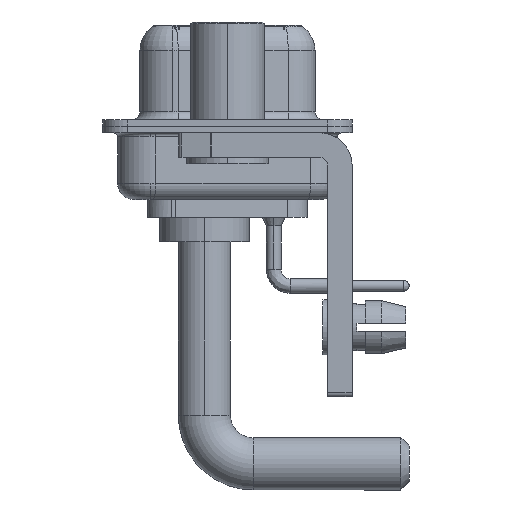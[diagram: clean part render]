
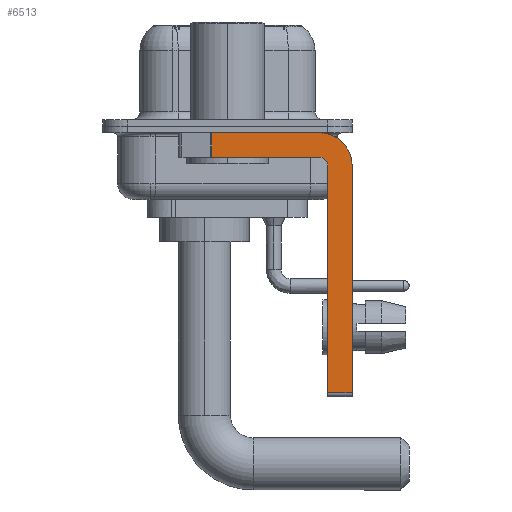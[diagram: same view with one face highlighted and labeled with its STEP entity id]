
A CAD part, left-side view. The second image highlights one B-rep face of the part: STEP entity #6513.
In plain terms, the highlighted planar face has unit normal (-1, 0, 0).
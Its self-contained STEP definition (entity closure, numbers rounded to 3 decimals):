
#29 = EDGE_CURVE ( 'NONE', #12476, #24220, #2890, .T. ) ;
#83 = DIRECTION ( 'NONE',  ( 0., 0., -1. ) ) ;
#709 = CARTESIAN_POINT ( 'NONE',  ( -2.9, -5.65, -0.4 ) ) ;
#879 = EDGE_CURVE ( 'NONE', #2302, #24220, #23438, .T. ) ;
#926 = AXIS2_PLACEMENT_3D ( 'NONE', #12614, #20422, #8382 ) ;
#1519 = DIRECTION ( 'NONE',  ( 1., 0., 0. ) ) ;
#1665 = LINE ( 'NONE', #15485, #15895 ) ;
#1714 = ORIENTED_EDGE ( 'NONE', *, *, #3956, .F. ) ;
#1825 = DIRECTION ( 'NONE',  ( 0., 0., 1. ) ) ;
#2302 = VERTEX_POINT ( 'NONE', #17210 ) ;
#2390 = ORIENTED_EDGE ( 'NONE', *, *, #879, .F. ) ;
#2756 = DIRECTION ( 'NONE',  ( 0., -1., 0. ) ) ;
#2890 = LINE ( 'NONE', #8523, #3668 ) ;
#3069 = PLANE ( 'NONE',  #11281 ) ;
#3343 = LINE ( 'NONE', #7564, #21656 ) ;
#3668 = VECTOR ( 'NONE', #2756, 1000. ) ;
#3956 = EDGE_CURVE ( 'NONE', #24719, #21280, #11832, .T. ) ;
#4261 = EDGE_CURVE ( 'NONE', #20301, #2302, #20989, .T. ) ;
#4277 = DIRECTION ( 'NONE',  ( 0., 1., 0. ) ) ;
#4703 = CARTESIAN_POINT ( 'NONE',  ( -2.9, -7.65, -16.35 ) ) ;
#4934 = CARTESIAN_POINT ( 'NONE',  ( -2.9, 3., -0.4 ) ) ;
#5697 = ORIENTED_EDGE ( 'NONE', *, *, #10876, .T. ) ;
#6239 = VECTOR ( 'NONE', #16693, 1000. ) ;
#6433 = CARTESIAN_POINT ( 'NONE',  ( -2.9, -6.15, -2.4 ) ) ;
#6513 = ADVANCED_FACE ( 'NONE', ( #8840 ), #3069, .F. ) ;
#6971 = CIRCLE ( 'NONE', #19246, 0.5 ) ;
#7502 = VECTOR ( 'NONE', #4277, 1000. ) ;
#7546 = ORIENTED_EDGE ( 'NONE', *, *, #16072, .F. ) ;
#7564 = CARTESIAN_POINT ( 'NONE',  ( -2.9, -6.15, -16.6 ) ) ;
#8382 = DIRECTION ( 'NONE',  ( 0., 0., -1. ) ) ;
#8523 = CARTESIAN_POINT ( 'NONE',  ( -2.9, -5.65, -16.35 ) ) ;
#8603 = ORIENTED_EDGE ( 'NONE', *, *, #16526, .F. ) ;
#8840 = FACE_OUTER_BOUND ( 'NONE', #10477, .T. ) ;
#8977 = DIRECTION ( 'NONE',  ( 0., 0., 1. ) ) ;
#10225 = CARTESIAN_POINT ( 'NONE',  ( -2.9, -7.65, -2.4 ) ) ;
#10477 = EDGE_LOOP ( 'NONE', ( #13567, #5697, #1714, #7546, #8603, #21376, #2390, #14541 ) ) ;
#10876 = EDGE_CURVE ( 'NONE', #15048, #21280, #1665, .T. ) ;
#11281 = AXIS2_PLACEMENT_3D ( 'NONE', #16771, #1519, #18954 ) ;
#11832 = LINE ( 'NONE', #13880, #7502 ) ;
#12405 = CARTESIAN_POINT ( 'NONE',  ( -2.9, 0.978, -0.4 ) ) ;
#12476 = VERTEX_POINT ( 'NONE', #13808 ) ;
#12614 = CARTESIAN_POINT ( 'NONE',  ( -2.9, -5.65, -2.4 ) ) ;
#13567 = ORIENTED_EDGE ( 'NONE', *, *, #19476, .F. ) ;
#13808 = CARTESIAN_POINT ( 'NONE',  ( -2.9, -6.15, -16.35 ) ) ;
#13880 = CARTESIAN_POINT ( 'NONE',  ( -2.9, -5.65, -1.9 ) ) ;
#14541 = ORIENTED_EDGE ( 'NONE', *, *, #4261, .F. ) ;
#14776 = LINE ( 'NONE', #4934, #6239 ) ;
#15048 = VERTEX_POINT ( 'NONE', #12405 ) ;
#15485 = CARTESIAN_POINT ( 'NONE',  ( -2.9, 0.978, -1.9 ) ) ;
#15895 = VECTOR ( 'NONE', #23444, 1000. ) ;
#16072 = EDGE_CURVE ( 'NONE', #21254, #24719, #6971, .T. ) ;
#16284 = CARTESIAN_POINT ( 'NONE',  ( -2.9, 0.978, -1.9 ) ) ;
#16526 = EDGE_CURVE ( 'NONE', #12476, #21254, #3343, .T. ) ;
#16693 = DIRECTION ( 'NONE',  ( 0., -1., 0. ) ) ;
#16771 = CARTESIAN_POINT ( 'NONE',  ( -2.9, -5.65, -2.4 ) ) ;
#17039 = CARTESIAN_POINT ( 'NONE',  ( -2.9, -5.65, -1.9 ) ) ;
#17062 = CARTESIAN_POINT ( 'NONE',  ( -2.9, -5.65, -2.4 ) ) ;
#17210 = CARTESIAN_POINT ( 'NONE',  ( -2.9, -7.65, -2.4 ) ) ;
#18954 = DIRECTION ( 'NONE',  ( 0., 0., -1. ) ) ;
#19246 = AXIS2_PLACEMENT_3D ( 'NONE', #17062, #21043, #1825 ) ;
#19476 = EDGE_CURVE ( 'NONE', #15048, #20301, #14776, .T. ) ;
#20301 = VERTEX_POINT ( 'NONE', #709 ) ;
#20422 = DIRECTION ( 'NONE',  ( 1., 0., 0. ) ) ;
#20989 = CIRCLE ( 'NONE', #926, 2. ) ;
#21043 = DIRECTION ( 'NONE',  ( -1., 0., 0. ) ) ;
#21254 = VERTEX_POINT ( 'NONE', #6433 ) ;
#21280 = VERTEX_POINT ( 'NONE', #16284 ) ;
#21376 = ORIENTED_EDGE ( 'NONE', *, *, #29, .T. ) ;
#21656 = VECTOR ( 'NONE', #8977, 1000. ) ;
#22611 = VECTOR ( 'NONE', #83, 1000. ) ;
#23438 = LINE ( 'NONE', #10225, #22611 ) ;
#23444 = DIRECTION ( 'NONE',  ( 0., 0., -1. ) ) ;
#24220 = VERTEX_POINT ( 'NONE', #4703 ) ;
#24719 = VERTEX_POINT ( 'NONE', #17039 ) ;
